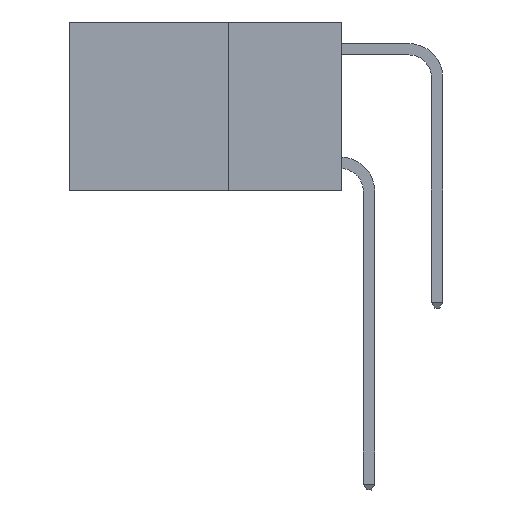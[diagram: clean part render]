
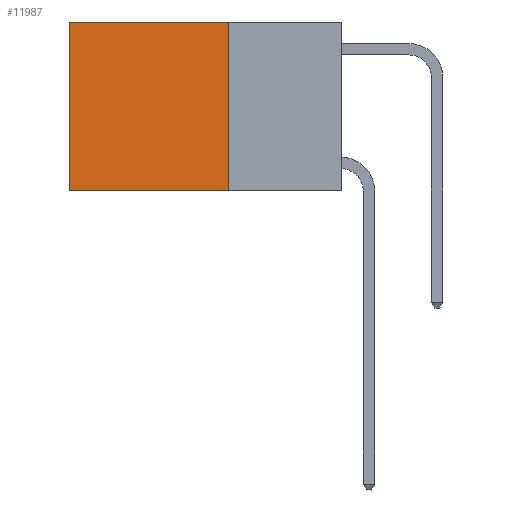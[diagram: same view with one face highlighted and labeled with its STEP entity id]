
A CAD part, left-side view. The second image highlights one B-rep face of the part: STEP entity #11987.
In plain terms, the highlighted planar face has unit normal (-1, 0, 0).
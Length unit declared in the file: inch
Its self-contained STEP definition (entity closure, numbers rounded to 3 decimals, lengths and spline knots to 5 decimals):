
#192 = DIRECTION ( 'NONE',  ( 0., 0., -1. ) ) ;
#772 = CARTESIAN_POINT ( 'NONE',  ( 0.2625, 0.25, 0. ) ) ;
#780 = AXIS2_PLACEMENT_3D ( 'NONE', #7461, #14670, #12190 ) ;
#1987 = VECTOR ( 'NONE', #14339, 39.37008 ) ;
#2478 = CARTESIAN_POINT ( 'NONE',  ( 0.2625, 0.25, -0.37 ) ) ;
#2557 = EDGE_CURVE ( 'NONE', #3988, #7499, #4766, .T. ) ;
#3245 = EDGE_LOOP ( 'NONE', ( #13429, #12756, #7182, #3461 ) ) ;
#3461 = ORIENTED_EDGE ( 'NONE', *, *, #12320, .T. ) ;
#3988 = VERTEX_POINT ( 'NONE', #11478 ) ;
#4402 = VERTEX_POINT ( 'NONE', #6573 ) ;
#4750 = PLANE ( 'NONE',  #780 ) ;
#4764 = VECTOR ( 'NONE', #14651, 39.37008 ) ;
#4766 = LINE ( 'NONE', #2478, #1987 ) ;
#4798 = CARTESIAN_POINT ( 'NONE',  ( 0.2625, 0.6, 0. ) ) ;
#5594 = EDGE_CURVE ( 'NONE', #4402, #7499, #11959, .T. ) ;
#6137 = CARTESIAN_POINT ( 'NONE',  ( 0.2625, 0.25, 0. ) ) ;
#6381 = FACE_OUTER_BOUND ( 'NONE', #3245, .T. ) ;
#6573 = CARTESIAN_POINT ( 'NONE',  ( 0.2625, 0.6, 0. ) ) ;
#7182 = ORIENTED_EDGE ( 'NONE', *, *, #11687, .F. ) ;
#7461 = CARTESIAN_POINT ( 'NONE',  ( 0.2625, 0.25, 0. ) ) ;
#7499 = VERTEX_POINT ( 'NONE', #10325 ) ;
#7887 = DIRECTION ( 'NONE',  ( 0., 0., -1. ) ) ;
#9417 = LINE ( 'NONE', #772, #9735 ) ;
#9735 = VECTOR ( 'NONE', #7887, 39.37008 ) ;
#9920 = LINE ( 'NONE', #6137, #4764 ) ;
#10325 = CARTESIAN_POINT ( 'NONE',  ( 0.2625, 0.6, -0.37 ) ) ;
#11212 = VECTOR ( 'NONE', #192, 39.37008 ) ;
#11478 = CARTESIAN_POINT ( 'NONE',  ( 0.2625, 0.25, -0.37 ) ) ;
#11687 = EDGE_CURVE ( 'NONE', #14749, #3988, #9417, .T. ) ;
#11959 = LINE ( 'NONE', #4798, #11212 ) ;
#11987 = ADVANCED_FACE ( 'NONE', ( #6381 ), #4750, .F. ) ;
#12190 = DIRECTION ( 'NONE',  ( 0., 0., -1. ) ) ;
#12294 = CARTESIAN_POINT ( 'NONE',  ( 0.2625, 0.25, 0. ) ) ;
#12320 = EDGE_CURVE ( 'NONE', #14749, #4402, #9920, .T. ) ;
#12756 = ORIENTED_EDGE ( 'NONE', *, *, #2557, .F. ) ;
#13429 = ORIENTED_EDGE ( 'NONE', *, *, #5594, .T. ) ;
#14339 = DIRECTION ( 'NONE',  ( 0., 1., 0. ) ) ;
#14651 = DIRECTION ( 'NONE',  ( 0., 1., 0. ) ) ;
#14670 = DIRECTION ( 'NONE',  ( 1., 0., 0. ) ) ;
#14749 = VERTEX_POINT ( 'NONE', #12294 ) ;
